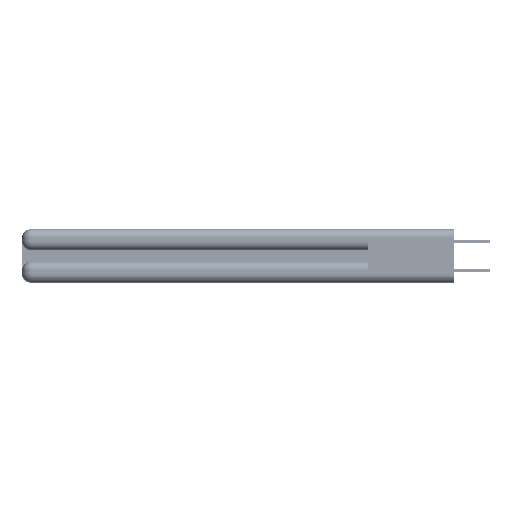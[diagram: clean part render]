
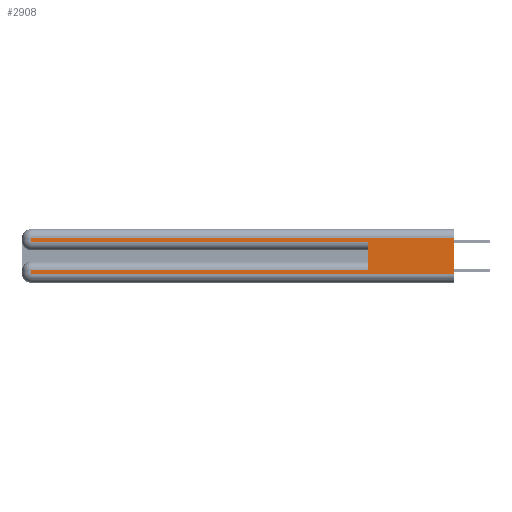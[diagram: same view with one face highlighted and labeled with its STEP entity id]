
A CAD part, left-side view. The second image highlights one B-rep face of the part: STEP entity #2908.
In plain terms, the highlighted planar face has unit normal (-1, 0, 0).
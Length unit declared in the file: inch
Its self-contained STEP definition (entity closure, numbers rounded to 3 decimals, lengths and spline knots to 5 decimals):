
#46 = VERTEX_POINT ( 'NONE', #35495 ) ;
#378 = CARTESIAN_POINT ( 'NONE',  ( 0., 2.94, 0.285 ) ) ;
#382 = CARTESIAN_POINT ( 'NONE',  ( 0., 0., 0.37 ) ) ;
#569 = ORIENTED_EDGE ( 'NONE', *, *, #5023, .T. ) ;
#1004 = EDGE_CURVE ( 'NONE', #8954, #38809, #28826, .T. ) ;
#1087 = CARTESIAN_POINT ( 'NONE',  ( 0., 0., 0.31 ) ) ;
#1342 = ORIENTED_EDGE ( 'NONE', *, *, #50269, .T. ) ;
#1435 = LINE ( 'NONE', #36614, #37781 ) ;
#2809 = VERTEX_POINT ( 'NONE', #49705 ) ;
#2908 = ADVANCED_FACE ( 'NONE', ( #18230 ), #42075, .F. ) ;
#3429 = DIRECTION ( 'NONE',  ( 0., 0., -1. ) ) ;
#5023 = EDGE_CURVE ( 'NONE', #20038, #42055, #11544, .T. ) ;
#6323 = VECTOR ( 'NONE', #31202, 39.37008 ) ;
#6362 = LINE ( 'NONE', #7215, #14739 ) ;
#7215 = CARTESIAN_POINT ( 'NONE',  ( 0., 2.94, 0.37 ) ) ;
#8954 = VERTEX_POINT ( 'NONE', #15461 ) ;
#11544 = LINE ( 'NONE', #39482, #6323 ) ;
#12380 = EDGE_CURVE ( 'NONE', #2809, #26083, #28298, .T. ) ;
#14326 = VECTOR ( 'NONE', #15392, 39.37008 ) ;
#14739 = VECTOR ( 'NONE', #19188, 39.37008 ) ;
#15392 = DIRECTION ( 'NONE',  ( 0., -1., 0. ) ) ;
#15461 = CARTESIAN_POINT ( 'NONE',  ( 0., 2.94, 0.31 ) ) ;
#16870 = DIRECTION ( 'NONE',  ( 0., -1., 0. ) ) ;
#17293 = EDGE_LOOP ( 'NONE', ( #34042, #44567, #24009, #1342, #42035, #569, #19887, #26390 ) ) ;
#18230 = FACE_OUTER_BOUND ( 'NONE', #17293, .T. ) ;
#19188 = DIRECTION ( 'NONE',  ( 0., 0., -1. ) ) ;
#19387 = CARTESIAN_POINT ( 'NONE',  ( 0., 0., 0.285 ) ) ;
#19887 = ORIENTED_EDGE ( 'NONE', *, *, #22667, .T. ) ;
#20038 = VERTEX_POINT ( 'NONE', #47310 ) ;
#21624 = DIRECTION ( 'NONE',  ( 1., 0., 0. ) ) ;
#22667 = EDGE_CURVE ( 'NONE', #42055, #2809, #6362, .T. ) ;
#22841 = LINE ( 'NONE', #48357, #53306 ) ;
#22941 = CARTESIAN_POINT ( 'NONE',  ( 0., 0.6, 0.285 ) ) ;
#24009 = ORIENTED_EDGE ( 'NONE', *, *, #1004, .T. ) ;
#26083 = VERTEX_POINT ( 'NONE', #47610 ) ;
#26390 = ORIENTED_EDGE ( 'NONE', *, *, #12380, .T. ) ;
#27668 = VECTOR ( 'NONE', #16870, 39.37008 ) ;
#27708 = DIRECTION ( 'NONE',  ( 0., 0., 1. ) ) ;
#28298 = LINE ( 'NONE', #41710, #27668 ) ;
#28826 = LINE ( 'NONE', #37039, #43065 ) ;
#30065 = VECTOR ( 'NONE', #30689, 39.37008 ) ;
#30689 = DIRECTION ( 'NONE',  ( 0., 1., 0. ) ) ;
#31202 = DIRECTION ( 'NONE',  ( 0., 1., 0. ) ) ;
#31381 = LINE ( 'NONE', #1087, #30065 ) ;
#33258 = DIRECTION ( 'NONE',  ( 0., 0., -1. ) ) ;
#33317 = AXIS2_PLACEMENT_3D ( 'NONE', #382, #21624, #42435 ) ;
#34042 = ORIENTED_EDGE ( 'NONE', *, *, #45975, .F. ) ;
#35422 = CARTESIAN_POINT ( 'NONE',  ( 0., 2.94, 0.085 ) ) ;
#35495 = CARTESIAN_POINT ( 'NONE',  ( 0., 0., 0.31 ) ) ;
#36055 = EDGE_CURVE ( 'NONE', #46, #8954, #31381, .T. ) ;
#36614 = CARTESIAN_POINT ( 'NONE',  ( 0., 0., 0.37 ) ) ;
#37039 = CARTESIAN_POINT ( 'NONE',  ( 0., 2.94, 0.37 ) ) ;
#37781 = VECTOR ( 'NONE', #3429, 39.37008 ) ;
#38809 = VERTEX_POINT ( 'NONE', #378 ) ;
#39482 = CARTESIAN_POINT ( 'NONE',  ( 0., 0., 0.085 ) ) ;
#41710 = CARTESIAN_POINT ( 'NONE',  ( 0., 0., 0.06 ) ) ;
#42025 = VERTEX_POINT ( 'NONE', #22941 ) ;
#42035 = ORIENTED_EDGE ( 'NONE', *, *, #49864, .F. ) ;
#42055 = VERTEX_POINT ( 'NONE', #35422 ) ;
#42075 = PLANE ( 'NONE',  #33317 ) ;
#42435 = DIRECTION ( 'NONE',  ( 0., 0., -1. ) ) ;
#43065 = VECTOR ( 'NONE', #33258, 39.37008 ) ;
#44567 = ORIENTED_EDGE ( 'NONE', *, *, #36055, .T. ) ;
#45509 = LINE ( 'NONE', #19387, #14326 ) ;
#45975 = EDGE_CURVE ( 'NONE', #46, #26083, #1435, .T. ) ;
#47310 = CARTESIAN_POINT ( 'NONE',  ( 0., 0.6, 0.085 ) ) ;
#47610 = CARTESIAN_POINT ( 'NONE',  ( 0., 0., 0.06 ) ) ;
#48357 = CARTESIAN_POINT ( 'NONE',  ( 0., 0.6, 0.145 ) ) ;
#49705 = CARTESIAN_POINT ( 'NONE',  ( 0., 2.94, 0.06 ) ) ;
#49864 = EDGE_CURVE ( 'NONE', #20038, #42025, #22841, .T. ) ;
#50269 = EDGE_CURVE ( 'NONE', #38809, #42025, #45509, .T. ) ;
#53306 = VECTOR ( 'NONE', #27708, 39.37008 ) ;
